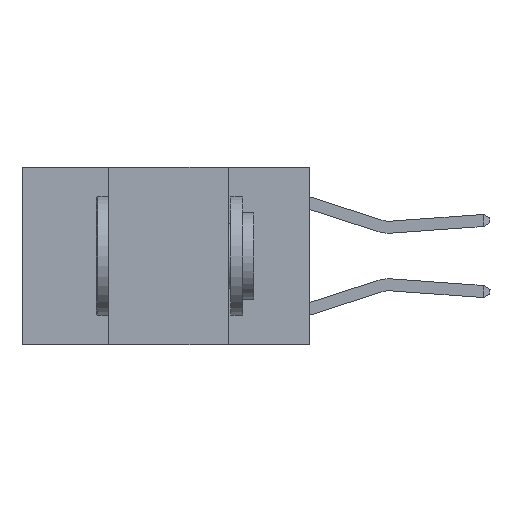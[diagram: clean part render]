
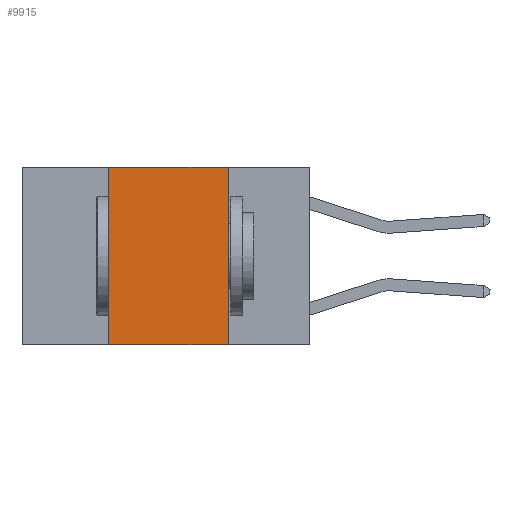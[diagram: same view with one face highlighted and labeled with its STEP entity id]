
A CAD part, left-side view. The second image highlights one B-rep face of the part: STEP entity #9915.
In plain terms, the highlighted planar face has unit normal (-1, 0, 0).
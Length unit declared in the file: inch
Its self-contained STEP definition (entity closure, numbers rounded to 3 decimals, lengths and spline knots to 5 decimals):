
#570 = CARTESIAN_POINT ( 'NONE',  ( 0., 0.17, -0.37 ) ) ;
#971 = EDGE_CURVE ( 'NONE', #1677, #3179, #23430, .T. ) ;
#1677 = VERTEX_POINT ( 'NONE', #3929 ) ;
#2366 = ORIENTED_EDGE ( 'NONE', *, *, #19923, .F. ) ;
#3039 = VECTOR ( 'NONE', #23629, 39.37008 ) ;
#3179 = VERTEX_POINT ( 'NONE', #570 ) ;
#3332 = CARTESIAN_POINT ( 'NONE',  ( 0., 0.42, 0. ) ) ;
#3929 = CARTESIAN_POINT ( 'NONE',  ( 0., 0.42, -0.37 ) ) ;
#4309 = CARTESIAN_POINT ( 'NONE',  ( 0., 0.6, -0.37 ) ) ;
#5129 = CARTESIAN_POINT ( 'NONE',  ( 0., 0.6, 0. ) ) ;
#6104 = EDGE_CURVE ( 'NONE', #1677, #17762, #9512, .T. ) ;
#6467 = ORIENTED_EDGE ( 'NONE', *, *, #25305, .F. ) ;
#8451 = AXIS2_PLACEMENT_3D ( 'NONE', #17492, #13112, #17894 ) ;
#9126 = VERTEX_POINT ( 'NONE', #16856 ) ;
#9512 = LINE ( 'NONE', #3332, #3039 ) ;
#9915 = ADVANCED_FACE ( 'NONE', ( #17638 ), #21483, .F. ) ;
#12090 = EDGE_LOOP ( 'NONE', ( #2366, #6467, #20025, #22952 ) ) ;
#13112 = DIRECTION ( 'NONE',  ( 1., 0., 0. ) ) ;
#16856 = CARTESIAN_POINT ( 'NONE',  ( 0., 0.17, 0. ) ) ;
#17492 = CARTESIAN_POINT ( 'NONE',  ( 0., 0.6, 0. ) ) ;
#17539 = DIRECTION ( 'NONE',  ( 0., 0., -1. ) ) ;
#17638 = FACE_OUTER_BOUND ( 'NONE', #12090, .T. ) ;
#17762 = VERTEX_POINT ( 'NONE', #21919 ) ;
#17894 = DIRECTION ( 'NONE',  ( 0., 0., -1. ) ) ;
#19886 = LINE ( 'NONE', #24288, #20252 ) ;
#19923 = EDGE_CURVE ( 'NONE', #9126, #3179, #19886, .T. ) ;
#20025 = ORIENTED_EDGE ( 'NONE', *, *, #6104, .F. ) ;
#20252 = VECTOR ( 'NONE', #17539, 39.37008 ) ;
#20843 = VECTOR ( 'NONE', #22040, 39.37008 ) ;
#21483 = PLANE ( 'NONE',  #8451 ) ;
#21919 = CARTESIAN_POINT ( 'NONE',  ( 0., 0.42, 0. ) ) ;
#22040 = DIRECTION ( 'NONE',  ( 0., -1., 0. ) ) ;
#22171 = LINE ( 'NONE', #5129, #20843 ) ;
#22866 = DIRECTION ( 'NONE',  ( 0., -1., 0. ) ) ;
#22952 = ORIENTED_EDGE ( 'NONE', *, *, #971, .T. ) ;
#23430 = LINE ( 'NONE', #4309, #23597 ) ;
#23597 = VECTOR ( 'NONE', #22866, 39.37008 ) ;
#23629 = DIRECTION ( 'NONE',  ( 0., 0., 1. ) ) ;
#24288 = CARTESIAN_POINT ( 'NONE',  ( 0., 0.17, 0. ) ) ;
#25305 = EDGE_CURVE ( 'NONE', #17762, #9126, #22171, .T. ) ;
